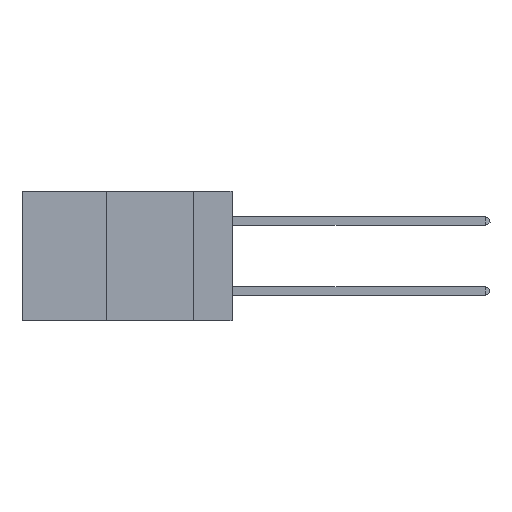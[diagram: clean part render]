
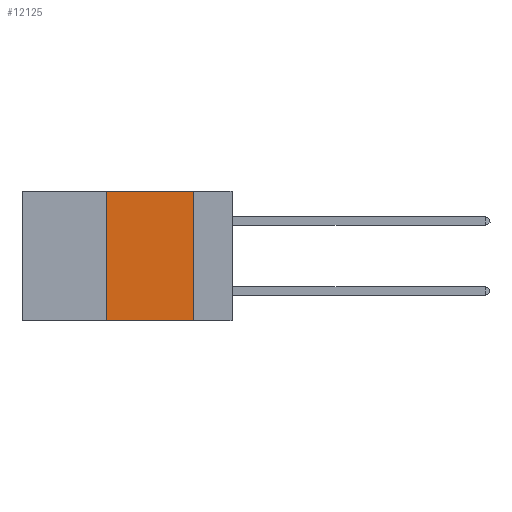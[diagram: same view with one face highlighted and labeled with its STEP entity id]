
A CAD part, left-side view. The second image highlights one B-rep face of the part: STEP entity #12125.
In plain terms, the highlighted planar face has unit normal (-1, 0, 0).
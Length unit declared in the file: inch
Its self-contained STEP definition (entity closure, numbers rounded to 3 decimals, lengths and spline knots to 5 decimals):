
#377 = CARTESIAN_POINT ( 'NONE',  ( 0., 0.11, 0. ) ) ;
#679 = ORIENTED_EDGE ( 'NONE', *, *, #12391, .F. ) ;
#1597 = LINE ( 'NONE', #21873, #17133 ) ;
#2841 = CARTESIAN_POINT ( 'NONE',  ( 0., 0.6, 0. ) ) ;
#3397 = VERTEX_POINT ( 'NONE', #377 ) ;
#3992 = CARTESIAN_POINT ( 'NONE',  ( 0., 0.6, 0. ) ) ;
#4283 = DIRECTION ( 'NONE',  ( 0., 0., 1. ) ) ;
#4389 = LINE ( 'NONE', #3992, #13281 ) ;
#4395 = DIRECTION ( 'NONE',  ( 1., 0., 0. ) ) ;
#4755 = EDGE_CURVE ( 'NONE', #17795, #9739, #1597, .T. ) ;
#4938 = VECTOR ( 'NONE', #6072, 39.37008 ) ;
#5054 = EDGE_CURVE ( 'NONE', #17795, #7526, #10971, .T. ) ;
#5492 = CARTESIAN_POINT ( 'NONE',  ( 0., 0.36, -0.37 ) ) ;
#6072 = DIRECTION ( 'NONE',  ( 0., 0., -1. ) ) ;
#7230 = ORIENTED_EDGE ( 'NONE', *, *, #11520, .F. ) ;
#7526 = VERTEX_POINT ( 'NONE', #16056 ) ;
#9244 = EDGE_LOOP ( 'NONE', ( #7230, #679, #11425, #21729 ) ) ;
#9739 = VERTEX_POINT ( 'NONE', #20366 ) ;
#9880 = PLANE ( 'NONE',  #11845 ) ;
#10971 = LINE ( 'NONE', #15306, #14915 ) ;
#11425 = ORIENTED_EDGE ( 'NONE', *, *, #4755, .F. ) ;
#11520 = EDGE_CURVE ( 'NONE', #3397, #7526, #19682, .T. ) ;
#11845 = AXIS2_PLACEMENT_3D ( 'NONE', #2841, #4395, #16808 ) ;
#12079 = DIRECTION ( 'NONE',  ( 0., -1., 0. ) ) ;
#12125 = ADVANCED_FACE ( 'NONE', ( #14660 ), #9880, .F. ) ;
#12391 = EDGE_CURVE ( 'NONE', #9739, #3397, #4389, .T. ) ;
#13281 = VECTOR ( 'NONE', #12079, 39.37008 ) ;
#14660 = FACE_OUTER_BOUND ( 'NONE', #9244, .T. ) ;
#14915 = VECTOR ( 'NONE', #15221, 39.37008 ) ;
#15221 = DIRECTION ( 'NONE',  ( 0., -1., 0. ) ) ;
#15306 = CARTESIAN_POINT ( 'NONE',  ( 0., 0.6, -0.37 ) ) ;
#16056 = CARTESIAN_POINT ( 'NONE',  ( 0., 0.11, -0.37 ) ) ;
#16716 = CARTESIAN_POINT ( 'NONE',  ( 0., 0.11, 0. ) ) ;
#16808 = DIRECTION ( 'NONE',  ( 0., 0., -1. ) ) ;
#17133 = VECTOR ( 'NONE', #4283, 39.37008 ) ;
#17795 = VERTEX_POINT ( 'NONE', #5492 ) ;
#19682 = LINE ( 'NONE', #16716, #4938 ) ;
#20366 = CARTESIAN_POINT ( 'NONE',  ( 0., 0.36, 0. ) ) ;
#21729 = ORIENTED_EDGE ( 'NONE', *, *, #5054, .T. ) ;
#21873 = CARTESIAN_POINT ( 'NONE',  ( 0., 0.36, 0. ) ) ;
